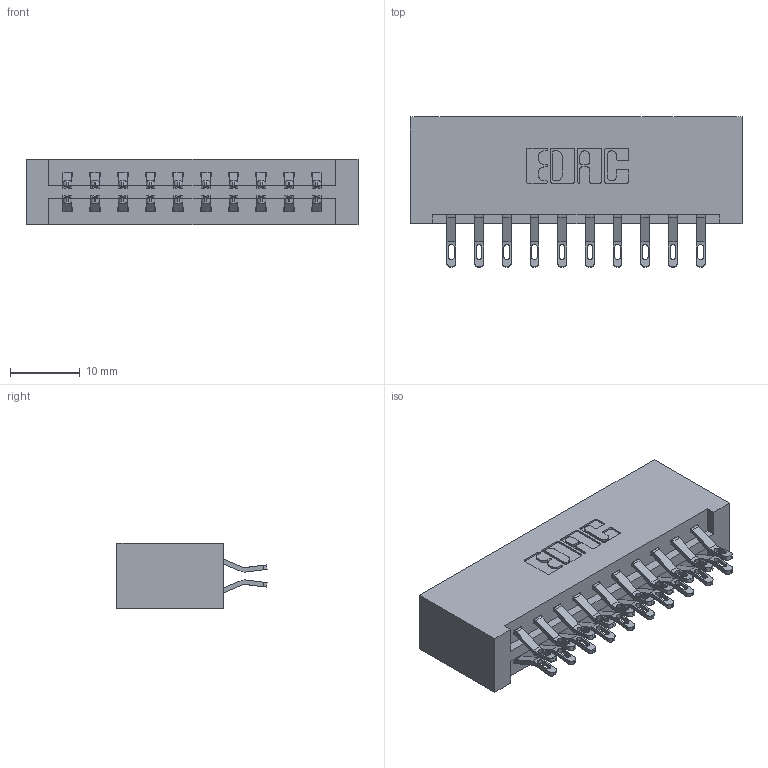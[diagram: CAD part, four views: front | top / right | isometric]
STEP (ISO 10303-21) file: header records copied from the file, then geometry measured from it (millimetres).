
FILE_DESCRIPTION (( 'STEP AP203' ), '1' );
FILE_NAME ('337-020-555-201.STEP', '2018-08-05T10:00:37', ( '' ), ( '' ), 'SwSTEP 2.0', 'SolidWorks 2016', '' );
FILE_SCHEMA (( 'CONFIG_CONTROL_DESIGN' ));
Length unit declared in the file: inch
Products named in the file (3): 337 Part_No Mounting Lugs; 345-292-001_555 Tail; 337-020-555-201
Assembly tree (21 placements, depth 2):
  337-020-555-201
    337 Part_No Mounting Lugs
    345-292-001_555 Tail  x20
Bounding box: 47.5 x 21.47 x 9.4 mm (x, y, z)
Volume: 5398.5 mm3; surface area: 6066.9 mm2
Topology: 21 solids, 21 shells, 1306 faces, 4067 edges, 2710 vertices
Faces by surface type: plane 786, cylinder 520
Entity records: 11941 total; most frequent: CARTESIAN_POINT 2072, ORIENTED_EDGE 1978, DIRECTION 1785, EDGE_CURVE 989, LINE 849, VECTOR 849, VERTEX_POINT 658, AXIS2_PLACEMENT_3D 468
